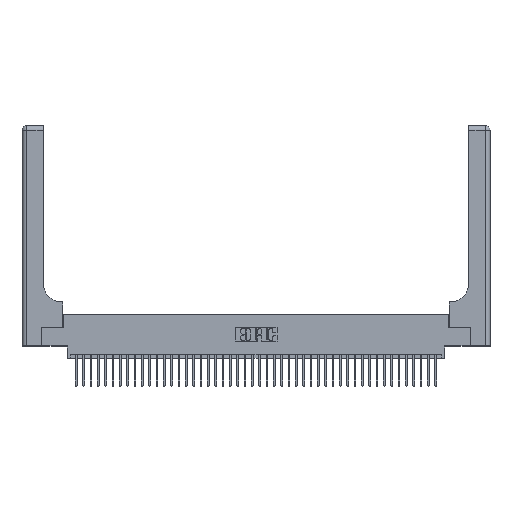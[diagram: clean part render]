
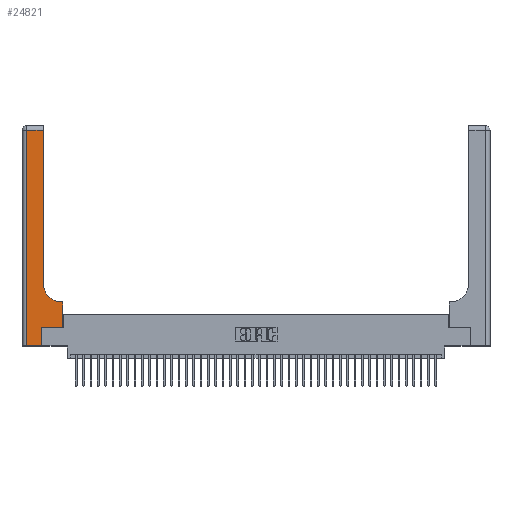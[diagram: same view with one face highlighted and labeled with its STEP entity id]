
A CAD part, top view. The second image highlights one B-rep face of the part: STEP entity #24821.
In plain terms, the highlighted planar face has unit normal (0, 0, 1).
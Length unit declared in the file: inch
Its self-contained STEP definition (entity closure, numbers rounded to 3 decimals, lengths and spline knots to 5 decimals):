
#238 = VERTEX_POINT ( 'NONE', #26446 ) ;
#859 = CARTESIAN_POINT ( 'NONE',  ( 0.2915, 0.85, 0.37 ) ) ;
#1012 = DIRECTION ( 'NONE',  ( 0., 0., -1. ) ) ;
#1131 = CARTESIAN_POINT ( 'NONE',  ( 0.5585, 0.25, 0.37 ) ) ;
#1202 = ORIENTED_EDGE ( 'NONE', *, *, #28185, .T. ) ;
#1810 = VECTOR ( 'NONE', #17673, 39.37008 ) ;
#1834 = VECTOR ( 'NONE', #3405, 39.37008 ) ;
#2468 = VECTOR ( 'NONE', #18234, 39.37008 ) ;
#2577 = CARTESIAN_POINT ( 'NONE',  ( 0.2915, 2.94, 0.37 ) ) ;
#3405 = DIRECTION ( 'NONE',  ( -1., 0., 0. ) ) ;
#4297 = CARTESIAN_POINT ( 'NONE',  ( 0.269, 0., 0.37 ) ) ;
#4908 = LINE ( 'NONE', #19335, #21844 ) ;
#5207 = VERTEX_POINT ( 'NONE', #29731 ) ;
#5664 = ORIENTED_EDGE ( 'NONE', *, *, #35942, .T. ) ;
#5849 = EDGE_CURVE ( 'NONE', #16142, #11703, #31953, .T. ) ;
#7707 = DIRECTION ( 'NONE',  ( 0., 1., 0. ) ) ;
#8813 = ORIENTED_EDGE ( 'NONE', *, *, #5849, .T. ) ;
#9373 = VECTOR ( 'NONE', #28177, 39.37008 ) ;
#10088 = DIRECTION ( 'NONE',  ( -1., 0., 0. ) ) ;
#11703 = VERTEX_POINT ( 'NONE', #859 ) ;
#12133 = LINE ( 'NONE', #4297, #28994 ) ;
#12293 = ORIENTED_EDGE ( 'NONE', *, *, #14961, .T. ) ;
#12554 = VERTEX_POINT ( 'NONE', #2577 ) ;
#14496 = CARTESIAN_POINT ( 'NONE',  ( 0., 3., 0.37 ) ) ;
#14961 = EDGE_CURVE ( 'NONE', #11703, #12554, #28756, .T. ) ;
#16142 = VERTEX_POINT ( 'NONE', #23769 ) ;
#16222 = VECTOR ( 'NONE', #10088, 39.37008 ) ;
#16388 = VERTEX_POINT ( 'NONE', #35987 ) ;
#17565 = EDGE_LOOP ( 'NONE', ( #12293, #40663, #43472, #17991, #5664, #42028, #41371, #1202, #8813 ) ) ;
#17673 = DIRECTION ( 'NONE',  ( 0., 1., 0. ) ) ;
#17976 = CARTESIAN_POINT ( 'NONE',  ( 0.5585, 0.25, 0.37 ) ) ;
#17991 = ORIENTED_EDGE ( 'NONE', *, *, #37928, .T. ) ;
#18234 = DIRECTION ( 'NONE',  ( 1., 0., 0. ) ) ;
#18750 = EDGE_CURVE ( 'NONE', #37166, #37567, #19432, .T. ) ;
#19335 = CARTESIAN_POINT ( 'NONE',  ( 0.06, 3., 0.37 ) ) ;
#19432 = LINE ( 'NONE', #1131, #9373 ) ;
#20031 = DIRECTION ( 'NONE',  ( 0., 0., -1. ) ) ;
#21071 = CARTESIAN_POINT ( 'NONE',  ( 0.2915, 3., 0.37 ) ) ;
#21311 = PLANE ( 'NONE',  #37734 ) ;
#21844 = VECTOR ( 'NONE', #42633, 39.37008 ) ;
#23082 = VECTOR ( 'NONE', #34448, 39.37008 ) ;
#23769 = CARTESIAN_POINT ( 'NONE',  ( 0.5415, 0.6, 0.37 ) ) ;
#23774 = AXIS2_PLACEMENT_3D ( 'NONE', #39981, #20031, #43322 ) ;
#24689 = DIRECTION ( 'NONE',  ( -1., 0., 0. ) ) ;
#24821 = ADVANCED_FACE ( 'NONE', ( #26698 ), #21311, .F. ) ;
#25291 = VERTEX_POINT ( 'NONE', #37040 ) ;
#26446 = CARTESIAN_POINT ( 'NONE',  ( 0.269, 0.25, 0.37 ) ) ;
#26698 = FACE_OUTER_BOUND ( 'NONE', #17565, .T. ) ;
#26876 = CARTESIAN_POINT ( 'NONE',  ( 0., 2.94, 0.37 ) ) ;
#27171 = CARTESIAN_POINT ( 'NONE',  ( 0.2915, 0.6, 0.37 ) ) ;
#27222 = EDGE_CURVE ( 'NONE', #5207, #16388, #4908, .T. ) ;
#28177 = DIRECTION ( 'NONE',  ( 0., 1., 0. ) ) ;
#28185 = EDGE_CURVE ( 'NONE', #37567, #16142, #42867, .T. ) ;
#28756 = LINE ( 'NONE', #21071, #1810 ) ;
#28994 = VECTOR ( 'NONE', #7707, 39.37008 ) ;
#29403 = LINE ( 'NONE', #31396, #2468 ) ;
#29731 = CARTESIAN_POINT ( 'NONE',  ( 0.06, 2.94, 0.37 ) ) ;
#30462 = EDGE_CURVE ( 'NONE', #238, #37166, #29403, .T. ) ;
#31090 = CARTESIAN_POINT ( 'NONE',  ( 0., 0., 0.37 ) ) ;
#31396 = CARTESIAN_POINT ( 'NONE',  ( 0.269, 0.25, 0.37 ) ) ;
#31953 = CIRCLE ( 'NONE', #23774, 0.25 ) ;
#32723 = CARTESIAN_POINT ( 'NONE',  ( 0.5585, 0.6, 0.37 ) ) ;
#32998 = LINE ( 'NONE', #31090, #23082 ) ;
#34448 = DIRECTION ( 'NONE',  ( 1., 0., 0. ) ) ;
#35942 = EDGE_CURVE ( 'NONE', #25291, #238, #12133, .T. ) ;
#35987 = CARTESIAN_POINT ( 'NONE',  ( 0.06, 0., 0.37 ) ) ;
#37040 = CARTESIAN_POINT ( 'NONE',  ( 0.269, 0., 0.37 ) ) ;
#37166 = VERTEX_POINT ( 'NONE', #17976 ) ;
#37567 = VERTEX_POINT ( 'NONE', #32723 ) ;
#37637 = LINE ( 'NONE', #26876, #1834 ) ;
#37734 = AXIS2_PLACEMENT_3D ( 'NONE', #14496, #1012, #24689 ) ;
#37751 = EDGE_CURVE ( 'NONE', #12554, #5207, #37637, .T. ) ;
#37928 = EDGE_CURVE ( 'NONE', #16388, #25291, #32998, .T. ) ;
#39981 = CARTESIAN_POINT ( 'NONE',  ( 0.5415, 0.85, 0.37 ) ) ;
#40663 = ORIENTED_EDGE ( 'NONE', *, *, #37751, .T. ) ;
#41371 = ORIENTED_EDGE ( 'NONE', *, *, #18750, .T. ) ;
#42028 = ORIENTED_EDGE ( 'NONE', *, *, #30462, .T. ) ;
#42633 = DIRECTION ( 'NONE',  ( 0., -1., 0. ) ) ;
#42867 = LINE ( 'NONE', #27171, #16222 ) ;
#43322 = DIRECTION ( 'NONE',  ( 1., 0., 0. ) ) ;
#43472 = ORIENTED_EDGE ( 'NONE', *, *, #27222, .T. ) ;
